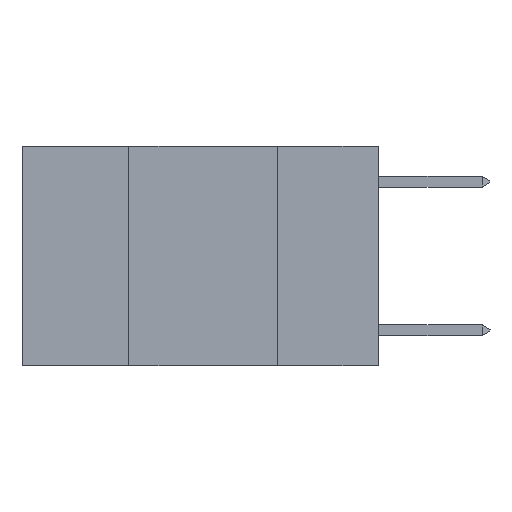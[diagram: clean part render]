
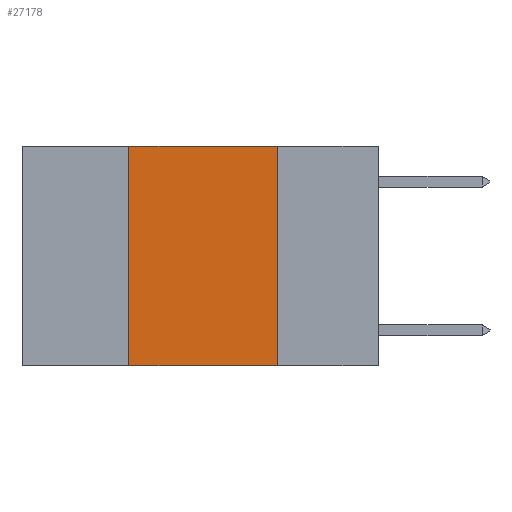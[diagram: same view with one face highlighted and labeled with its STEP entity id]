
A CAD part, left-side view. The second image highlights one B-rep face of the part: STEP entity #27178.
In plain terms, the highlighted planar face has unit normal (-1, 0, 0).
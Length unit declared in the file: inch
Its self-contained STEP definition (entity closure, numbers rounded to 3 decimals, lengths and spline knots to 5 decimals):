
#256 = FACE_OUTER_BOUND ( 'NONE', #22144, .T. ) ;
#536 = CARTESIAN_POINT ( 'NONE',  ( 0., 0.6, 0. ) ) ;
#2140 = CARTESIAN_POINT ( 'NONE',  ( 0., 0.42, -0.37 ) ) ;
#2793 = DIRECTION ( 'NONE',  ( 0., -1., 0. ) ) ;
#3070 = LINE ( 'NONE', #19879, #15754 ) ;
#4426 = CARTESIAN_POINT ( 'NONE',  ( 0., 0.17, 0. ) ) ;
#5527 = EDGE_CURVE ( 'NONE', #7418, #11251, #3070, .T. ) ;
#6198 = DIRECTION ( 'NONE',  ( 0., 0., 1. ) ) ;
#6280 = CARTESIAN_POINT ( 'NONE',  ( 0., 0.6, -0.37 ) ) ;
#6455 = CARTESIAN_POINT ( 'NONE',  ( 0., 0.17, -0.37 ) ) ;
#6931 = DIRECTION ( 'NONE',  ( 0., 0., -1. ) ) ;
#7418 = VERTEX_POINT ( 'NONE', #24105 ) ;
#8010 = ORIENTED_EDGE ( 'NONE', *, *, #5527, .F. ) ;
#10455 = AXIS2_PLACEMENT_3D ( 'NONE', #536, #26427, #6931 ) ;
#10574 = LINE ( 'NONE', #6280, #18266 ) ;
#10781 = CARTESIAN_POINT ( 'NONE',  ( 0., 0.42, 0. ) ) ;
#10858 = VERTEX_POINT ( 'NONE', #2140 ) ;
#11251 = VERTEX_POINT ( 'NONE', #17968 ) ;
#12878 = EDGE_CURVE ( 'NONE', #11251, #21553, #28061, .T. ) ;
#12960 = EDGE_CURVE ( 'NONE', #10858, #21553, #10574, .T. ) ;
#14836 = DIRECTION ( 'NONE',  ( 0., -1., 0. ) ) ;
#15430 = VECTOR ( 'NONE', #6198, 39.37008 ) ;
#15754 = VECTOR ( 'NONE', #2793, 39.37008 ) ;
#17229 = VECTOR ( 'NONE', #24070, 39.37008 ) ;
#17315 = LINE ( 'NONE', #10781, #15430 ) ;
#17610 = PLANE ( 'NONE',  #10455 ) ;
#17968 = CARTESIAN_POINT ( 'NONE',  ( 0., 0.17, 0. ) ) ;
#18266 = VECTOR ( 'NONE', #14836, 39.37008 ) ;
#19879 = CARTESIAN_POINT ( 'NONE',  ( 0., 0.6, 0. ) ) ;
#20428 = ORIENTED_EDGE ( 'NONE', *, *, #12960, .T. ) ;
#21485 = ORIENTED_EDGE ( 'NONE', *, *, #23034, .F. ) ;
#21553 = VERTEX_POINT ( 'NONE', #6455 ) ;
#22144 = EDGE_LOOP ( 'NONE', ( #25700, #8010, #21485, #20428 ) ) ;
#23034 = EDGE_CURVE ( 'NONE', #10858, #7418, #17315, .T. ) ;
#24070 = DIRECTION ( 'NONE',  ( 0., 0., -1. ) ) ;
#24105 = CARTESIAN_POINT ( 'NONE',  ( 0., 0.42, 0. ) ) ;
#25700 = ORIENTED_EDGE ( 'NONE', *, *, #12878, .F. ) ;
#26427 = DIRECTION ( 'NONE',  ( 1., 0., 0. ) ) ;
#27178 = ADVANCED_FACE ( 'NONE', ( #256 ), #17610, .F. ) ;
#28061 = LINE ( 'NONE', #4426, #17229 ) ;
